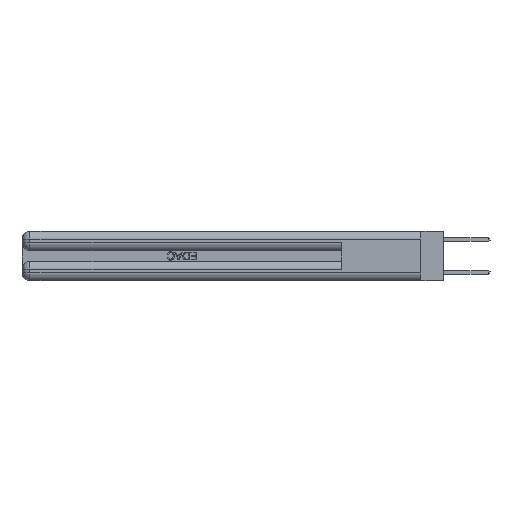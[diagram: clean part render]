
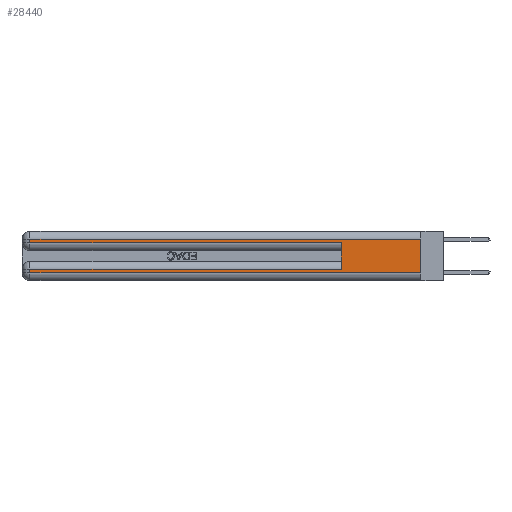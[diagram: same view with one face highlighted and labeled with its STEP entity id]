
A CAD part, left-side view. The second image highlights one B-rep face of the part: STEP entity #28440.
In plain terms, the highlighted planar face has unit normal (-1, 0, 0).
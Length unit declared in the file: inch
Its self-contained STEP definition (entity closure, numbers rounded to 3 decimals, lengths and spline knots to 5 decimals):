
#104 = EDGE_CURVE ( 'NONE', #10893, #14974, #6383, .T. ) ;
#196 = VECTOR ( 'NONE', #18846, 39.37008 ) ;
#200 = VERTEX_POINT ( 'NONE', #16467 ) ;
#230 = DIRECTION ( 'NONE',  ( 1., 0., 0. ) ) ;
#347 = CARTESIAN_POINT ( 'NONE',  ( 0., 0., 0.37 ) ) ;
#396 = DIRECTION ( 'NONE',  ( 0., -1., 0. ) ) ;
#642 = VERTEX_POINT ( 'NONE', #10898 ) ;
#724 = CARTESIAN_POINT ( 'NONE',  ( 0., 0., 0.06 ) ) ;
#749 = EDGE_CURVE ( 'NONE', #28988, #642, #2438, .T. ) ;
#1046 = LINE ( 'NONE', #28629, #16701 ) ;
#1273 = CARTESIAN_POINT ( 'NONE',  ( 0., 2.94, 0.31 ) ) ;
#1621 = VECTOR ( 'NONE', #29475, 39.37008 ) ;
#2438 = LINE ( 'NONE', #24907, #34097 ) ;
#2537 = EDGE_CURVE ( 'NONE', #34199, #642, #25568, .T. ) ;
#3129 = VERTEX_POINT ( 'NONE', #9183 ) ;
#4980 = VERTEX_POINT ( 'NONE', #1273 ) ;
#5359 = CARTESIAN_POINT ( 'NONE',  ( 0., 0., 0.31 ) ) ;
#6051 = CARTESIAN_POINT ( 'NONE',  ( 0., 2.94, 0.37 ) ) ;
#6383 = LINE ( 'NONE', #347, #25844 ) ;
#7204 = CARTESIAN_POINT ( 'NONE',  ( 0., 0., 0.085 ) ) ;
#7767 = CARTESIAN_POINT ( 'NONE',  ( 0., 0., 0.37 ) ) ;
#8109 = ORIENTED_EDGE ( 'NONE', *, *, #749, .T. ) ;
#8258 = LINE ( 'NONE', #25577, #14484 ) ;
#9183 = CARTESIAN_POINT ( 'NONE',  ( 0., 2.94, 0.085 ) ) ;
#10893 = VERTEX_POINT ( 'NONE', #5359 ) ;
#10898 = CARTESIAN_POINT ( 'NONE',  ( 0., 0.6, 0.285 ) ) ;
#11559 = EDGE_CURVE ( 'NONE', #34199, #3129, #35171, .T. ) ;
#11930 = DIRECTION ( 'NONE',  ( 0., 0., -1. ) ) ;
#12269 = DIRECTION ( 'NONE',  ( 0., -1., 0. ) ) ;
#14024 = PLANE ( 'NONE',  #14139 ) ;
#14139 = AXIS2_PLACEMENT_3D ( 'NONE', #7767, #230, #19217 ) ;
#14484 = VECTOR ( 'NONE', #30740, 39.37008 ) ;
#14868 = EDGE_CURVE ( 'NONE', #10893, #4980, #8258, .T. ) ;
#14974 = VERTEX_POINT ( 'NONE', #724 ) ;
#15898 = CARTESIAN_POINT ( 'NONE',  ( 0., 0.6, 0.085 ) ) ;
#15904 = ORIENTED_EDGE ( 'NONE', *, *, #35788, .T. ) ;
#15976 = ORIENTED_EDGE ( 'NONE', *, *, #104, .F. ) ;
#16171 = EDGE_CURVE ( 'NONE', #3129, #200, #31643, .T. ) ;
#16467 = CARTESIAN_POINT ( 'NONE',  ( 0., 2.94, 0.06 ) ) ;
#16701 = VECTOR ( 'NONE', #12269, 39.37008 ) ;
#17721 = CARTESIAN_POINT ( 'NONE',  ( 0., 2.94, 0.37 ) ) ;
#18191 = ORIENTED_EDGE ( 'NONE', *, *, #26303, .T. ) ;
#18347 = VECTOR ( 'NONE', #28138, 39.37008 ) ;
#18846 = DIRECTION ( 'NONE',  ( 0., 1., 0. ) ) ;
#19217 = DIRECTION ( 'NONE',  ( 0., 0., -1. ) ) ;
#19301 = VECTOR ( 'NONE', #25956, 39.37008 ) ;
#24907 = CARTESIAN_POINT ( 'NONE',  ( 0., 0., 0.285 ) ) ;
#25524 = EDGE_LOOP ( 'NONE', ( #15976, #28935, #15904, #8109, #26514, #33036, #36224, #18191 ) ) ;
#25568 = LINE ( 'NONE', #33463, #18347 ) ;
#25577 = CARTESIAN_POINT ( 'NONE',  ( 0., 0., 0.31 ) ) ;
#25844 = VECTOR ( 'NONE', #11930, 39.37008 ) ;
#25956 = DIRECTION ( 'NONE',  ( 0., 0., -1. ) ) ;
#26303 = EDGE_CURVE ( 'NONE', #200, #14974, #1046, .T. ) ;
#26514 = ORIENTED_EDGE ( 'NONE', *, *, #2537, .F. ) ;
#26535 = LINE ( 'NONE', #17721, #1621 ) ;
#28138 = DIRECTION ( 'NONE',  ( 0., 0., 1. ) ) ;
#28440 = ADVANCED_FACE ( 'NONE', ( #32979 ), #14024, .F. ) ;
#28629 = CARTESIAN_POINT ( 'NONE',  ( 0., 0., 0.06 ) ) ;
#28935 = ORIENTED_EDGE ( 'NONE', *, *, #14868, .T. ) ;
#28988 = VERTEX_POINT ( 'NONE', #34017 ) ;
#29475 = DIRECTION ( 'NONE',  ( 0., 0., -1. ) ) ;
#30740 = DIRECTION ( 'NONE',  ( 0., 1., 0. ) ) ;
#31643 = LINE ( 'NONE', #6051, #19301 ) ;
#32979 = FACE_OUTER_BOUND ( 'NONE', #25524, .T. ) ;
#33036 = ORIENTED_EDGE ( 'NONE', *, *, #11559, .T. ) ;
#33463 = CARTESIAN_POINT ( 'NONE',  ( 0., 0.6, 0.145 ) ) ;
#34017 = CARTESIAN_POINT ( 'NONE',  ( 0., 2.94, 0.285 ) ) ;
#34097 = VECTOR ( 'NONE', #396, 39.37008 ) ;
#34199 = VERTEX_POINT ( 'NONE', #15898 ) ;
#35171 = LINE ( 'NONE', #7204, #196 ) ;
#35788 = EDGE_CURVE ( 'NONE', #4980, #28988, #26535, .T. ) ;
#36224 = ORIENTED_EDGE ( 'NONE', *, *, #16171, .T. ) ;
